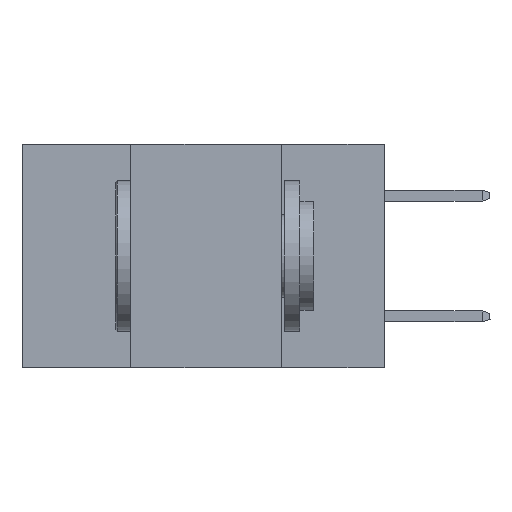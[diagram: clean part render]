
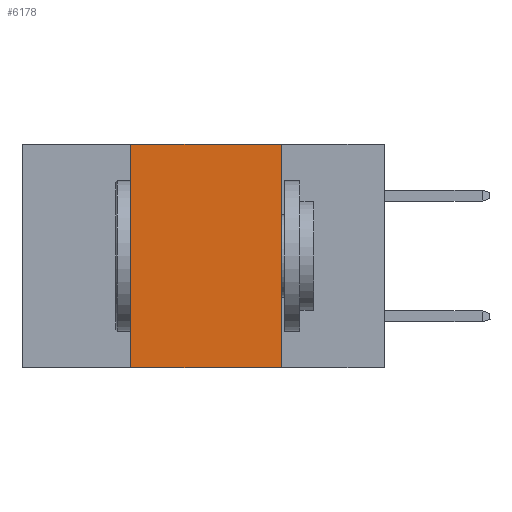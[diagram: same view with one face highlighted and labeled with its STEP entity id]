
A CAD part, left-side view. The second image highlights one B-rep face of the part: STEP entity #6178.
In plain terms, the highlighted planar face has unit normal (-1, 0, 0).
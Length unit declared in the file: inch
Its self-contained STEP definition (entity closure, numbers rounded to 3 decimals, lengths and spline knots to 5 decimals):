
#1693 = VECTOR ( 'NONE', #24330, 39.37008 ) ;
#2395 = EDGE_CURVE ( 'NONE', #25709, #21698, #12237, .T. ) ;
#3593 = VERTEX_POINT ( 'NONE', #15688 ) ;
#3958 = ORIENTED_EDGE ( 'NONE', *, *, #19546, .F. ) ;
#4561 = VECTOR ( 'NONE', #13904, 39.37008 ) ;
#4796 = CARTESIAN_POINT ( 'NONE',  ( 0., 0.6, 0. ) ) ;
#5340 = AXIS2_PLACEMENT_3D ( 'NONE', #4796, #22554, #7414 ) ;
#6178 = ADVANCED_FACE ( 'NONE', ( #6817 ), #7310, .F. ) ;
#6207 = CARTESIAN_POINT ( 'NONE',  ( 0., 0.17, -0.37 ) ) ;
#6817 = FACE_OUTER_BOUND ( 'NONE', #28849, .T. ) ;
#7310 = PLANE ( 'NONE',  #5340 ) ;
#7414 = DIRECTION ( 'NONE',  ( 0., 0., -1. ) ) ;
#9414 = LINE ( 'NONE', #21797, #1693 ) ;
#9999 = LINE ( 'NONE', #28421, #15958 ) ;
#10633 = CARTESIAN_POINT ( 'NONE',  ( 0., 0.6, 0. ) ) ;
#12237 = LINE ( 'NONE', #10633, #4561 ) ;
#12798 = EDGE_CURVE ( 'NONE', #3593, #16598, #9999, .T. ) ;
#13904 = DIRECTION ( 'NONE',  ( 0., -1., 0. ) ) ;
#15449 = EDGE_CURVE ( 'NONE', #3593, #25709, #9414, .T. ) ;
#15688 = CARTESIAN_POINT ( 'NONE',  ( 0., 0.42, -0.37 ) ) ;
#15958 = VECTOR ( 'NONE', #30934, 39.37008 ) ;
#16598 = VERTEX_POINT ( 'NONE', #6207 ) ;
#16706 = LINE ( 'NONE', #19235, #29233 ) ;
#17591 = ORIENTED_EDGE ( 'NONE', *, *, #2395, .F. ) ;
#19135 = ORIENTED_EDGE ( 'NONE', *, *, #15449, .F. ) ;
#19235 = CARTESIAN_POINT ( 'NONE',  ( 0., 0.17, 0. ) ) ;
#19546 = EDGE_CURVE ( 'NONE', #21698, #16598, #16706, .T. ) ;
#21698 = VERTEX_POINT ( 'NONE', #24656 ) ;
#21797 = CARTESIAN_POINT ( 'NONE',  ( 0., 0.42, 0. ) ) ;
#22554 = DIRECTION ( 'NONE',  ( 1., 0., 0. ) ) ;
#23794 = CARTESIAN_POINT ( 'NONE',  ( 0., 0.42, 0. ) ) ;
#24330 = DIRECTION ( 'NONE',  ( 0., 0., 1. ) ) ;
#24656 = CARTESIAN_POINT ( 'NONE',  ( 0., 0.17, 0. ) ) ;
#25709 = VERTEX_POINT ( 'NONE', #23794 ) ;
#25818 = ORIENTED_EDGE ( 'NONE', *, *, #12798, .T. ) ;
#26786 = DIRECTION ( 'NONE',  ( 0., 0., -1. ) ) ;
#28421 = CARTESIAN_POINT ( 'NONE',  ( 0., 0.6, -0.37 ) ) ;
#28849 = EDGE_LOOP ( 'NONE', ( #3958, #17591, #19135, #25818 ) ) ;
#29233 = VECTOR ( 'NONE', #26786, 39.37008 ) ;
#30934 = DIRECTION ( 'NONE',  ( 0., -1., 0. ) ) ;
